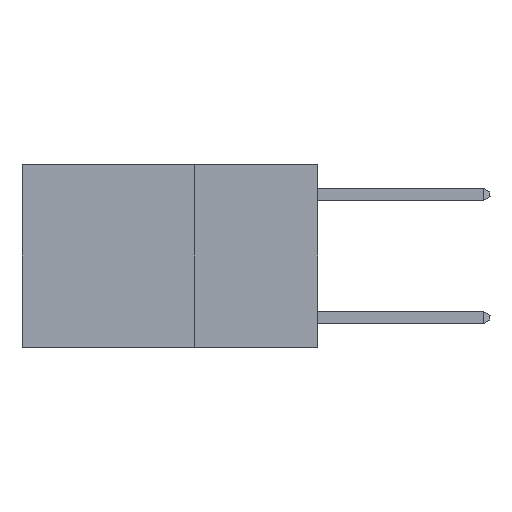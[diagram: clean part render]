
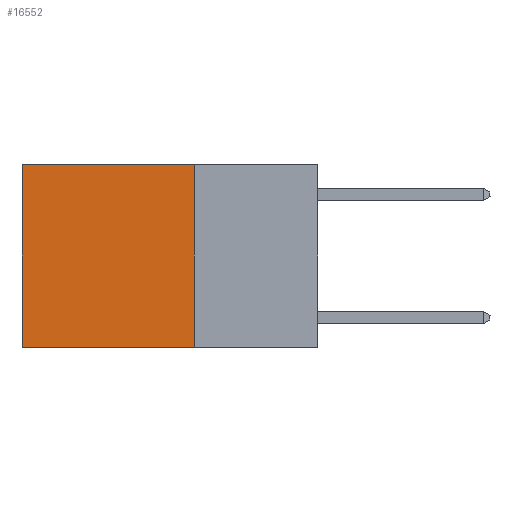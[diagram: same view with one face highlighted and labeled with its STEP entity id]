
A CAD part, left-side view. The second image highlights one B-rep face of the part: STEP entity #16552.
In plain terms, the highlighted planar face has unit normal (-1, 0, 0).
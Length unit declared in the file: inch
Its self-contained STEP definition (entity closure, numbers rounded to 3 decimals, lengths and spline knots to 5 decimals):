
#644 = CARTESIAN_POINT ( 'NONE',  ( 0.2625, 0.25, 0. ) ) ;
#709 = VERTEX_POINT ( 'NONE', #12068 ) ;
#1338 = ORIENTED_EDGE ( 'NONE', *, *, #13522, .T. ) ;
#1714 = VECTOR ( 'NONE', #13665, 39.37008 ) ;
#2671 = EDGE_CURVE ( 'NONE', #9012, #18274, #17922, .T. ) ;
#3465 = DIRECTION ( 'NONE',  ( 0., 0., -1. ) ) ;
#4427 = EDGE_CURVE ( 'NONE', #13811, #709, #4809, .T. ) ;
#4751 = DIRECTION ( 'NONE',  ( 0., 1., 0. ) ) ;
#4809 = LINE ( 'NONE', #11759, #16263 ) ;
#5112 = DIRECTION ( 'NONE',  ( 1., 0., 0. ) ) ;
#5425 = AXIS2_PLACEMENT_3D ( 'NONE', #18013, #5112, #9462 ) ;
#5541 = LINE ( 'NONE', #15122, #1714 ) ;
#6317 = LINE ( 'NONE', #644, #9207 ) ;
#9012 = VERTEX_POINT ( 'NONE', #14453 ) ;
#9207 = VECTOR ( 'NONE', #3465, 39.37008 ) ;
#9391 = DIRECTION ( 'NONE',  ( 0., 1., 0. ) ) ;
#9462 = DIRECTION ( 'NONE',  ( 0., 0., -1. ) ) ;
#10763 = ORIENTED_EDGE ( 'NONE', *, *, #11676, .F. ) ;
#11374 = ORIENTED_EDGE ( 'NONE', *, *, #2671, .T. ) ;
#11469 = ORIENTED_EDGE ( 'NONE', *, *, #4427, .F. ) ;
#11676 = EDGE_CURVE ( 'NONE', #9012, #13811, #6317, .T. ) ;
#11721 = FACE_OUTER_BOUND ( 'NONE', #12297, .T. ) ;
#11759 = CARTESIAN_POINT ( 'NONE',  ( 0.2625, 0.25, -0.37 ) ) ;
#12068 = CARTESIAN_POINT ( 'NONE',  ( 0.2625, 0.6, -0.37 ) ) ;
#12297 = EDGE_LOOP ( 'NONE', ( #1338, #11469, #10763, #11374 ) ) ;
#13522 = EDGE_CURVE ( 'NONE', #18274, #709, #5541, .T. ) ;
#13665 = DIRECTION ( 'NONE',  ( 0., 0., -1. ) ) ;
#13811 = VERTEX_POINT ( 'NONE', #17034 ) ;
#14453 = CARTESIAN_POINT ( 'NONE',  ( 0.2625, 0.25, 0. ) ) ;
#14743 = CARTESIAN_POINT ( 'NONE',  ( 0.2625, 0.25, 0. ) ) ;
#15122 = CARTESIAN_POINT ( 'NONE',  ( 0.2625, 0.6, 0. ) ) ;
#15174 = VECTOR ( 'NONE', #9391, 39.37008 ) ;
#15600 = CARTESIAN_POINT ( 'NONE',  ( 0.2625, 0.6, 0. ) ) ;
#16263 = VECTOR ( 'NONE', #4751, 39.37008 ) ;
#16552 = ADVANCED_FACE ( 'NONE', ( #11721 ), #16558, .F. ) ;
#16558 = PLANE ( 'NONE',  #5425 ) ;
#17034 = CARTESIAN_POINT ( 'NONE',  ( 0.2625, 0.25, -0.37 ) ) ;
#17922 = LINE ( 'NONE', #14743, #15174 ) ;
#18013 = CARTESIAN_POINT ( 'NONE',  ( 0.2625, 0.25, 0. ) ) ;
#18274 = VERTEX_POINT ( 'NONE', #15600 ) ;
